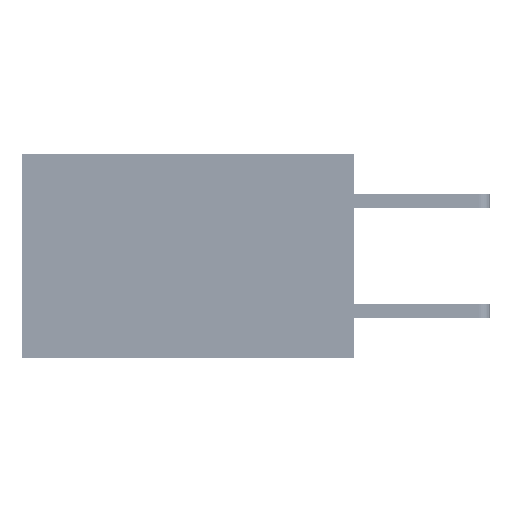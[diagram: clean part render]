
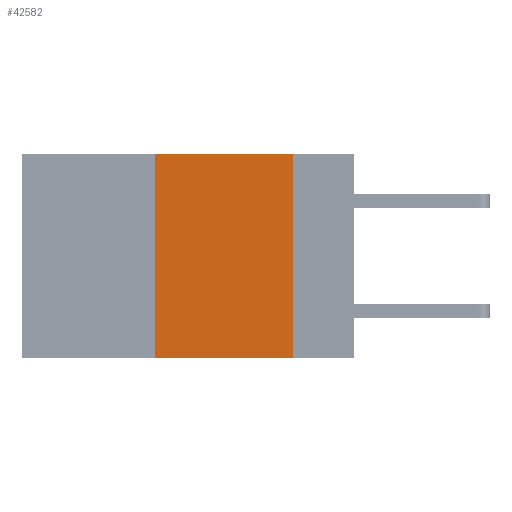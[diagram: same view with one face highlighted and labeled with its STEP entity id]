
A CAD part, left-side view. The second image highlights one B-rep face of the part: STEP entity #42582.
In plain terms, the highlighted planar face has unit normal (-1, 0, 0).
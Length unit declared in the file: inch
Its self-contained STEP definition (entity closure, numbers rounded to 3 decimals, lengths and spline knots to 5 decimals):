
#286 = CARTESIAN_POINT ( 'NONE',  ( 0., 0.6, -0.37 ) ) ;
#1576 = EDGE_CURVE ( 'NONE', #1876, #1657, #22467, .T. ) ;
#1657 = VERTEX_POINT ( 'NONE', #40785 ) ;
#1855 = ORIENTED_EDGE ( 'NONE', *, *, #11883, .F. ) ;
#1876 = VERTEX_POINT ( 'NONE', #39281 ) ;
#4389 = DIRECTION ( 'NONE',  ( 1., 0., 0. ) ) ;
#6922 = EDGE_LOOP ( 'NONE', ( #1855, #24242, #44069, #37046 ) ) ;
#7753 = DIRECTION ( 'NONE',  ( 0., -1., 0. ) ) ;
#8110 = PLANE ( 'NONE',  #21568 ) ;
#11098 = LINE ( 'NONE', #286, #35539 ) ;
#11871 = CARTESIAN_POINT ( 'NONE',  ( 0., 0.36, -0.37 ) ) ;
#11883 = EDGE_CURVE ( 'NONE', #1657, #47047, #18539, .T. ) ;
#13783 = VECTOR ( 'NONE', #29805, 39.37008 ) ;
#15017 = DIRECTION ( 'NONE',  ( 0., -1., 0. ) ) ;
#15225 = EDGE_CURVE ( 'NONE', #37378, #1876, #16657, .T. ) ;
#16657 = LINE ( 'NONE', #31605, #46403 ) ;
#18539 = LINE ( 'NONE', #33468, #13783 ) ;
#19147 = CARTESIAN_POINT ( 'NONE',  ( 0., 0.6, 0. ) ) ;
#21568 = AXIS2_PLACEMENT_3D ( 'NONE', #19147, #4389, #23071 ) ;
#22467 = LINE ( 'NONE', #41297, #39034 ) ;
#23071 = DIRECTION ( 'NONE',  ( 0., 0., -1. ) ) ;
#24242 = ORIENTED_EDGE ( 'NONE', *, *, #1576, .F. ) ;
#26320 = CARTESIAN_POINT ( 'NONE',  ( 0., 0.11, -0.37 ) ) ;
#26987 = FACE_OUTER_BOUND ( 'NONE', #6922, .T. ) ;
#29805 = DIRECTION ( 'NONE',  ( 0., 0., -1. ) ) ;
#31605 = CARTESIAN_POINT ( 'NONE',  ( 0., 0.36, 0. ) ) ;
#33468 = CARTESIAN_POINT ( 'NONE',  ( 0., 0.11, 0. ) ) ;
#35539 = VECTOR ( 'NONE', #15017, 39.37008 ) ;
#37046 = ORIENTED_EDGE ( 'NONE', *, *, #47118, .T. ) ;
#37378 = VERTEX_POINT ( 'NONE', #11871 ) ;
#39034 = VECTOR ( 'NONE', #7753, 39.37008 ) ;
#39281 = CARTESIAN_POINT ( 'NONE',  ( 0., 0.36, 0. ) ) ;
#40785 = CARTESIAN_POINT ( 'NONE',  ( 0., 0.11, 0. ) ) ;
#41297 = CARTESIAN_POINT ( 'NONE',  ( 0., 0.6, 0. ) ) ;
#42582 = ADVANCED_FACE ( 'NONE', ( #26987 ), #8110, .F. ) ;
#42845 = DIRECTION ( 'NONE',  ( 0., 0., 1. ) ) ;
#44069 = ORIENTED_EDGE ( 'NONE', *, *, #15225, .F. ) ;
#46403 = VECTOR ( 'NONE', #42845, 39.37008 ) ;
#47047 = VERTEX_POINT ( 'NONE', #26320 ) ;
#47118 = EDGE_CURVE ( 'NONE', #37378, #47047, #11098, .T. ) ;
